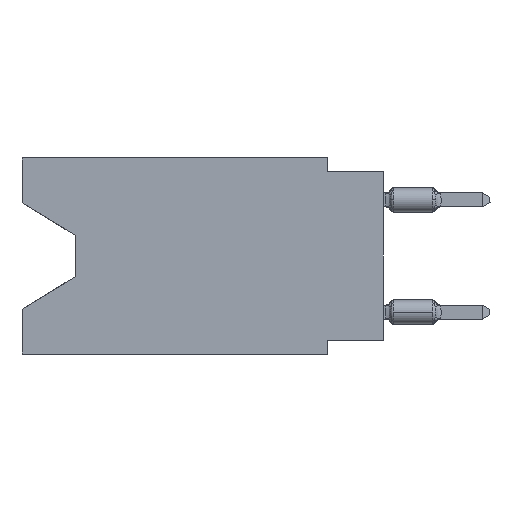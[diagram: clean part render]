
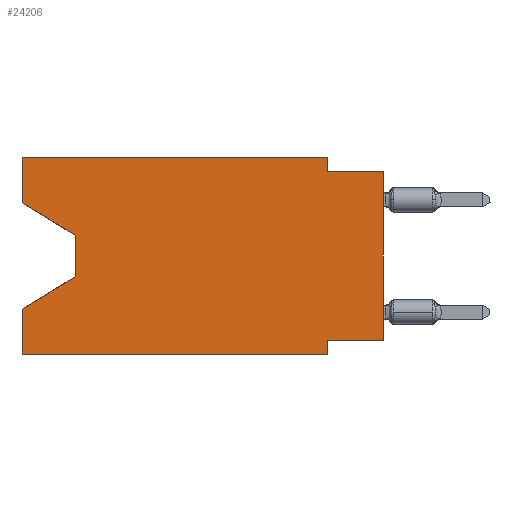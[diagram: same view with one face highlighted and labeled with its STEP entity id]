
A CAD part, left-side view. The second image highlights one B-rep face of the part: STEP entity #24206.
In plain terms, the highlighted planar face has unit normal (-1, 0, 0).
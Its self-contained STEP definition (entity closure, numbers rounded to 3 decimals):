
#102 = ORIENTED_EDGE ( 'NONE', *, *, #8468, .F. ) ;
#451 = EDGE_CURVE ( 'NONE', #9377, #23838, #10060, .T. ) ;
#469 = CARTESIAN_POINT ( 'NONE',  ( 0., 2.54, 0. ) ) ;
#506 = VECTOR ( 'NONE', #7865, 1000. ) ;
#619 = EDGE_LOOP ( 'NONE', ( #6738, #22676, #2506, #6275, #12986, #9600, #14710, #19012, #9160, #1234, #14886, #102 ) ) ;
#967 = EDGE_CURVE ( 'NONE', #9377, #7547, #16713, .T. ) ;
#1234 = ORIENTED_EDGE ( 'NONE', *, *, #20569, .F. ) ;
#1265 = CARTESIAN_POINT ( 'NONE',  ( 0., 16.383, 0. ) ) ;
#1301 = CARTESIAN_POINT ( 'NONE',  ( 0., 13.97, -3.505 ) ) ;
#1563 = CARTESIAN_POINT ( 'NONE',  ( 0., 16.383, -2.038 ) ) ;
#1663 = VERTEX_POINT ( 'NONE', #1301 ) ;
#1753 = VECTOR ( 'NONE', #4402, 1000. ) ;
#2101 = EDGE_CURVE ( 'NONE', #8785, #3104, #19189, .T. ) ;
#2415 = CARTESIAN_POINT ( 'NONE',  ( 0., 13.97, -5.385 ) ) ;
#2506 = ORIENTED_EDGE ( 'NONE', *, *, #22859, .T. ) ;
#2775 = CARTESIAN_POINT ( 'NONE',  ( 0., 0., -0.635 ) ) ;
#3104 = VERTEX_POINT ( 'NONE', #22983 ) ;
#3255 = CARTESIAN_POINT ( 'NONE',  ( 0., 13.97, -3.505 ) ) ;
#3640 = DIRECTION ( 'NONE',  ( 0., 0., 1. ) ) ;
#3919 = CARTESIAN_POINT ( 'NONE',  ( 0., 0., 0. ) ) ;
#4306 = EDGE_CURVE ( 'NONE', #1663, #20193, #20470, .T. ) ;
#4402 = DIRECTION ( 'NONE',  ( 0., -1., 0. ) ) ;
#4942 = EDGE_CURVE ( 'NONE', #14987, #1663, #8007, .T. ) ;
#5185 = VECTOR ( 'NONE', #8980, 1000. ) ;
#5214 = EDGE_CURVE ( 'NONE', #3104, #23838, #18628, .T. ) ;
#5505 = CARTESIAN_POINT ( 'NONE',  ( 0., 0., -8.255 ) ) ;
#5534 = EDGE_CURVE ( 'NONE', #12555, #24529, #19710, .T. ) ;
#5673 = VECTOR ( 'NONE', #7109, 1000. ) ;
#5766 = CARTESIAN_POINT ( 'NONE',  ( 0., 0., -8.255 ) ) ;
#6275 = ORIENTED_EDGE ( 'NONE', *, *, #967, .F. ) ;
#6599 = EDGE_CURVE ( 'NONE', #24792, #8570, #10516, .T. ) ;
#6738 = ORIENTED_EDGE ( 'NONE', *, *, #4942, .T. ) ;
#7109 = DIRECTION ( 'NONE',  ( 0., 0., -1. ) ) ;
#7547 = VERTEX_POINT ( 'NONE', #16387 ) ;
#7562 = CARTESIAN_POINT ( 'NONE',  ( 0., 16.383, 0. ) ) ;
#7671 = VECTOR ( 'NONE', #19285, 1000. ) ;
#7865 = DIRECTION ( 'NONE',  ( 0., 0.855, -0.519 ) ) ;
#7911 = DIRECTION ( 'NONE',  ( 0., 1., 0. ) ) ;
#8007 = LINE ( 'NONE', #15730, #7671 ) ;
#8220 = VECTOR ( 'NONE', #8738, 1000. ) ;
#8304 = VECTOR ( 'NONE', #3640, 1000. ) ;
#8468 = EDGE_CURVE ( 'NONE', #14987, #24792, #20982, .T. ) ;
#8497 = AXIS2_PLACEMENT_3D ( 'NONE', #14437, #22172, #16205 ) ;
#8570 = VERTEX_POINT ( 'NONE', #469 ) ;
#8656 = DIRECTION ( 'NONE',  ( 0., -1., 0. ) ) ;
#8738 = DIRECTION ( 'NONE',  ( 0., 0., -1. ) ) ;
#8785 = VERTEX_POINT ( 'NONE', #5505 ) ;
#8980 = DIRECTION ( 'NONE',  ( 0., -1., 0. ) ) ;
#9160 = ORIENTED_EDGE ( 'NONE', *, *, #5534, .F. ) ;
#9377 = VERTEX_POINT ( 'NONE', #10392 ) ;
#9600 = ORIENTED_EDGE ( 'NONE', *, *, #5214, .F. ) ;
#9711 = CARTESIAN_POINT ( 'NONE',  ( 0., 16.383, 0. ) ) ;
#10060 = LINE ( 'NONE', #24098, #10120 ) ;
#10120 = VECTOR ( 'NONE', #8656, 1000. ) ;
#10392 = CARTESIAN_POINT ( 'NONE',  ( 0., 16.383, -8.89 ) ) ;
#10516 = LINE ( 'NONE', #1265, #5185 ) ;
#10765 = PLANE ( 'NONE',  #8497 ) ;
#11168 = CARTESIAN_POINT ( 'NONE',  ( 0., 2.54, -8.89 ) ) ;
#11631 = VECTOR ( 'NONE', #18748, 1000. ) ;
#12555 = VERTEX_POINT ( 'NONE', #18716 ) ;
#12986 = ORIENTED_EDGE ( 'NONE', *, *, #451, .T. ) ;
#13767 = VECTOR ( 'NONE', #15682, 1000. ) ;
#13896 = CARTESIAN_POINT ( 'NONE',  ( 0., 0., -0.635 ) ) ;
#14036 = LINE ( 'NONE', #3919, #13767 ) ;
#14198 = LINE ( 'NONE', #18366, #8220 ) ;
#14437 = CARTESIAN_POINT ( 'NONE',  ( 0., 16.383, 0. ) ) ;
#14703 = CARTESIAN_POINT ( 'NONE',  ( 0., 2.54, -8.89 ) ) ;
#14710 = ORIENTED_EDGE ( 'NONE', *, *, #2101, .F. ) ;
#14886 = ORIENTED_EDGE ( 'NONE', *, *, #6599, .F. ) ;
#14987 = VERTEX_POINT ( 'NONE', #1563 ) ;
#15682 = DIRECTION ( 'NONE',  ( 0., 0., 1. ) ) ;
#15730 = CARTESIAN_POINT ( 'NONE',  ( 0., 16.383, -2.038 ) ) ;
#16205 = DIRECTION ( 'NONE',  ( 0., 0., -1. ) ) ;
#16387 = CARTESIAN_POINT ( 'NONE',  ( 0., 16.383, -6.852 ) ) ;
#16403 = DIRECTION ( 'NONE',  ( 0., 0., -1. ) ) ;
#16713 = LINE ( 'NONE', #24191, #11631 ) ;
#16860 = CARTESIAN_POINT ( 'NONE',  ( 0., 13.97, -5.385 ) ) ;
#17321 = VECTOR ( 'NONE', #7911, 1000. ) ;
#18043 = VECTOR ( 'NONE', #16403, 1000. ) ;
#18366 = CARTESIAN_POINT ( 'NONE',  ( 0., 2.54, 0. ) ) ;
#18628 = LINE ( 'NONE', #14703, #5673 ) ;
#18716 = CARTESIAN_POINT ( 'NONE',  ( 0., 2.54, -0.635 ) ) ;
#18748 = DIRECTION ( 'NONE',  ( 0., 0., 1. ) ) ;
#19012 = ORIENTED_EDGE ( 'NONE', *, *, #24429, .T. ) ;
#19189 = LINE ( 'NONE', #5766, #17321 ) ;
#19285 = DIRECTION ( 'NONE',  ( 0., -0.855, -0.519 ) ) ;
#19710 = LINE ( 'NONE', #13896, #1753 ) ;
#20193 = VERTEX_POINT ( 'NONE', #16860 ) ;
#20470 = LINE ( 'NONE', #3255, #18043 ) ;
#20569 = EDGE_CURVE ( 'NONE', #8570, #12555, #14198, .T. ) ;
#20982 = LINE ( 'NONE', #9711, #8304 ) ;
#22172 = DIRECTION ( 'NONE',  ( 1., 0., 0. ) ) ;
#22676 = ORIENTED_EDGE ( 'NONE', *, *, #4306, .T. ) ;
#22859 = EDGE_CURVE ( 'NONE', #20193, #7547, #23559, .T. ) ;
#22983 = CARTESIAN_POINT ( 'NONE',  ( 0., 2.54, -8.255 ) ) ;
#23559 = LINE ( 'NONE', #2415, #506 ) ;
#23838 = VERTEX_POINT ( 'NONE', #11168 ) ;
#24066 = FACE_OUTER_BOUND ( 'NONE', #619, .T. ) ;
#24098 = CARTESIAN_POINT ( 'NONE',  ( 0., 16.383, -8.89 ) ) ;
#24191 = CARTESIAN_POINT ( 'NONE',  ( 0., 16.383, 0. ) ) ;
#24206 = ADVANCED_FACE ( 'NONE', ( #24066 ), #10765, .F. ) ;
#24429 = EDGE_CURVE ( 'NONE', #8785, #24529, #14036, .T. ) ;
#24529 = VERTEX_POINT ( 'NONE', #2775 ) ;
#24792 = VERTEX_POINT ( 'NONE', #7562 ) ;
